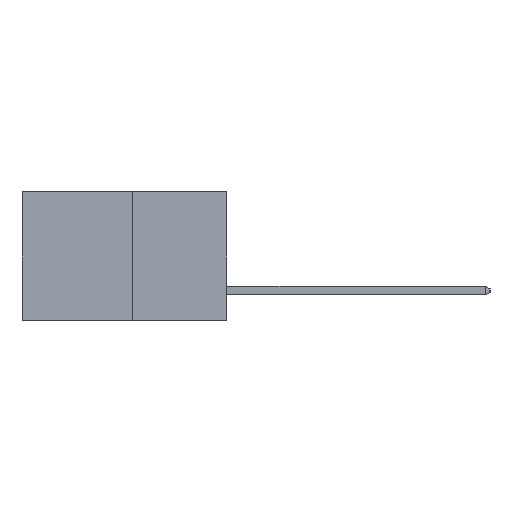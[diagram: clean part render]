
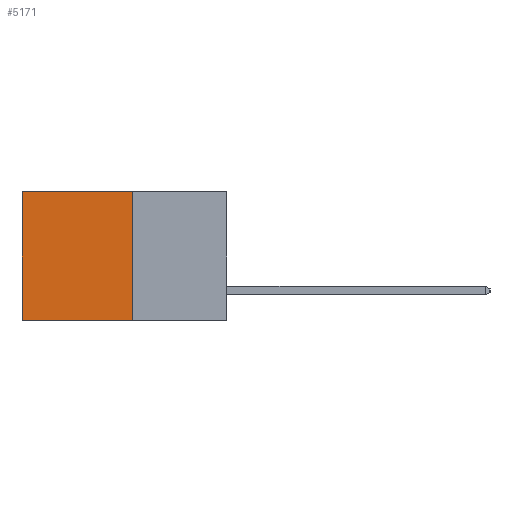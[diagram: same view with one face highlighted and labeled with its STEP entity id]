
A CAD part, left-side view. The second image highlights one B-rep face of the part: STEP entity #5171.
In plain terms, the highlighted planar face has unit normal (-1, 0, 0).
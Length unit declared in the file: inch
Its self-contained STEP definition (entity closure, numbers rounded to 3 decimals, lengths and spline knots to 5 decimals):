
#251 = VECTOR ( 'NONE', #8166, 39.37008 ) ;
#1463 = CARTESIAN_POINT ( 'NONE',  ( 0.277, 0.27, -0.37 ) ) ;
#1632 = VERTEX_POINT ( 'NONE', #7502 ) ;
#1721 = EDGE_CURVE ( 'NONE', #1632, #1834, #4542, .T. ) ;
#1834 = VERTEX_POINT ( 'NONE', #4366 ) ;
#1985 = EDGE_CURVE ( 'NONE', #1632, #4734, #2465, .T. ) ;
#2045 = LINE ( 'NONE', #7570, #10060 ) ;
#2053 = EDGE_CURVE ( 'NONE', #4734, #8249, #8480, .T. ) ;
#2073 = DIRECTION ( 'NONE',  ( 0., 0., -1. ) ) ;
#2465 = LINE ( 'NONE', #6628, #251 ) ;
#3259 = ORIENTED_EDGE ( 'NONE', *, *, #1721, .F. ) ;
#3872 = CARTESIAN_POINT ( 'NONE',  ( 0.277, 0.59, -0.37 ) ) ;
#4366 = CARTESIAN_POINT ( 'NONE',  ( 0.277, 0.27, -0.37 ) ) ;
#4542 = LINE ( 'NONE', #1463, #8365 ) ;
#4734 = VERTEX_POINT ( 'NONE', #8920 ) ;
#5082 = ORIENTED_EDGE ( 'NONE', *, *, #1985, .T. ) ;
#5171 = ADVANCED_FACE ( 'NONE', ( #7751 ), #6203, .F. ) ;
#6132 = DIRECTION ( 'NONE',  ( 0., 0., -1. ) ) ;
#6144 = DIRECTION ( 'NONE',  ( 1., 0., 0. ) ) ;
#6155 = CARTESIAN_POINT ( 'NONE',  ( 0.277, 0.27, -0.37 ) ) ;
#6203 = PLANE ( 'NONE',  #8239 ) ;
#6325 = EDGE_LOOP ( 'NONE', ( #8951, #7186, #3259, #5082 ) ) ;
#6628 = CARTESIAN_POINT ( 'NONE',  ( 0.277, 0.27, 0. ) ) ;
#7186 = ORIENTED_EDGE ( 'NONE', *, *, #9939, .F. ) ;
#7502 = CARTESIAN_POINT ( 'NONE',  ( 0.277, 0.27, 0. ) ) ;
#7570 = CARTESIAN_POINT ( 'NONE',  ( 0.277, 0.27, -0.37 ) ) ;
#7751 = FACE_OUTER_BOUND ( 'NONE', #6325, .T. ) ;
#8021 = VECTOR ( 'NONE', #9887, 39.37008 ) ;
#8166 = DIRECTION ( 'NONE',  ( 0., 1., 0. ) ) ;
#8239 = AXIS2_PLACEMENT_3D ( 'NONE', #6155, #6144, #6132 ) ;
#8249 = VERTEX_POINT ( 'NONE', #9281 ) ;
#8365 = VECTOR ( 'NONE', #2073, 39.37008 ) ;
#8480 = LINE ( 'NONE', #3872, #8021 ) ;
#8920 = CARTESIAN_POINT ( 'NONE',  ( 0.277, 0.59, 0. ) ) ;
#8951 = ORIENTED_EDGE ( 'NONE', *, *, #2053, .T. ) ;
#9053 = DIRECTION ( 'NONE',  ( 0., 1., 0. ) ) ;
#9281 = CARTESIAN_POINT ( 'NONE',  ( 0.277, 0.59, -0.37 ) ) ;
#9887 = DIRECTION ( 'NONE',  ( 0., 0., -1. ) ) ;
#9939 = EDGE_CURVE ( 'NONE', #1834, #8249, #2045, .T. ) ;
#10060 = VECTOR ( 'NONE', #9053, 39.37008 ) ;
